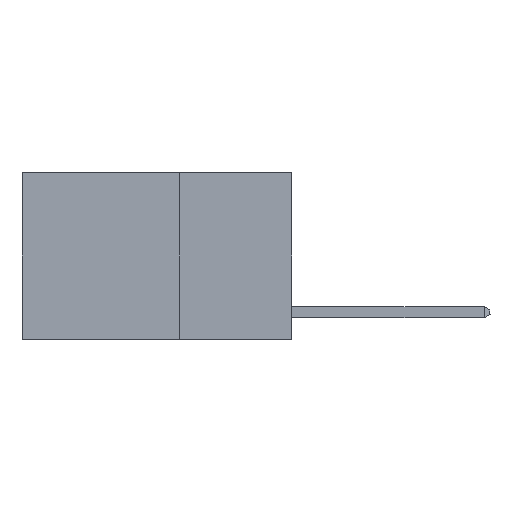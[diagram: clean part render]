
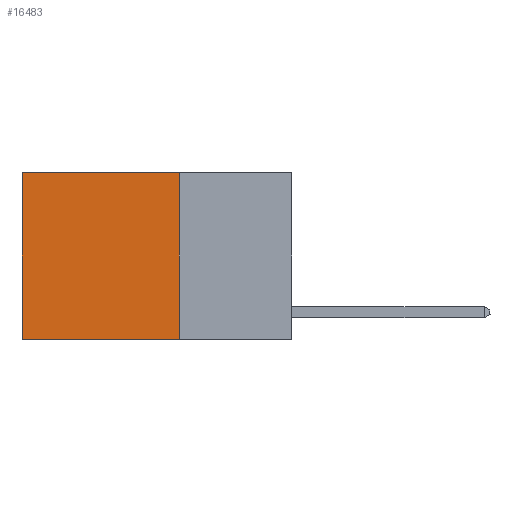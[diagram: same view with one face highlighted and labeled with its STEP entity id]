
A CAD part, left-side view. The second image highlights one B-rep face of the part: STEP entity #16483.
In plain terms, the highlighted planar face has unit normal (-1, 0, 0).
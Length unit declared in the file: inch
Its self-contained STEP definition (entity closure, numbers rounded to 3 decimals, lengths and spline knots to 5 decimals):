
#211 = DIRECTION ( 'NONE',  ( 0., 0., -1. ) ) ;
#755 = CARTESIAN_POINT ( 'NONE',  ( 0.2625, 0.25, -0.37 ) ) ;
#944 = CARTESIAN_POINT ( 'NONE',  ( 0.2625, 0.25, 0. ) ) ;
#2361 = LINE ( 'NONE', #10757, #10748 ) ;
#2517 = CARTESIAN_POINT ( 'NONE',  ( 0.2625, 0.25, 0. ) ) ;
#3203 = EDGE_CURVE ( 'NONE', #7254, #12237, #17413, .T. ) ;
#3739 = DIRECTION ( 'NONE',  ( 0., 0., -1. ) ) ;
#4208 = DIRECTION ( 'NONE',  ( 0., 0., -1. ) ) ;
#6625 = ORIENTED_EDGE ( 'NONE', *, *, #14745, .T. ) ;
#7254 = VERTEX_POINT ( 'NONE', #7407 ) ;
#7407 = CARTESIAN_POINT ( 'NONE',  ( 0.2625, 0.6, 0. ) ) ;
#8365 = VERTEX_POINT ( 'NONE', #944 ) ;
#8452 = VECTOR ( 'NONE', #14415, 39.37008 ) ;
#8497 = EDGE_LOOP ( 'NONE', ( #17888, #10391, #9834, #6625 ) ) ;
#9010 = VECTOR ( 'NONE', #3739, 39.37008 ) ;
#9834 = ORIENTED_EDGE ( 'NONE', *, *, #10853, .F. ) ;
#10391 = ORIENTED_EDGE ( 'NONE', *, *, #19052, .F. ) ;
#10748 = VECTOR ( 'NONE', #14100, 39.37008 ) ;
#10757 = CARTESIAN_POINT ( 'NONE',  ( 0.2625, 0.25, 0. ) ) ;
#10853 = EDGE_CURVE ( 'NONE', #8365, #15404, #19815, .T. ) ;
#11202 = FACE_OUTER_BOUND ( 'NONE', #8497, .T. ) ;
#12237 = VERTEX_POINT ( 'NONE', #15357 ) ;
#14100 = DIRECTION ( 'NONE',  ( 0., 1., 0. ) ) ;
#14223 = DIRECTION ( 'NONE',  ( 1., 0., 0. ) ) ;
#14415 = DIRECTION ( 'NONE',  ( 0., 1., 0. ) ) ;
#14745 = EDGE_CURVE ( 'NONE', #8365, #7254, #2361, .T. ) ;
#15357 = CARTESIAN_POINT ( 'NONE',  ( 0.2625, 0.6, -0.37 ) ) ;
#15404 = VERTEX_POINT ( 'NONE', #755 ) ;
#15450 = CARTESIAN_POINT ( 'NONE',  ( 0.2625, 0.6, 0. ) ) ;
#16483 = ADVANCED_FACE ( 'NONE', ( #11202 ), #20955, .F. ) ;
#17358 = LINE ( 'NONE', #19449, #8452 ) ;
#17413 = LINE ( 'NONE', #15450, #9010 ) ;
#17888 = ORIENTED_EDGE ( 'NONE', *, *, #3203, .T. ) ;
#18514 = AXIS2_PLACEMENT_3D ( 'NONE', #2517, #14223, #4208 ) ;
#19052 = EDGE_CURVE ( 'NONE', #15404, #12237, #17358, .T. ) ;
#19281 = VECTOR ( 'NONE', #211, 39.37008 ) ;
#19449 = CARTESIAN_POINT ( 'NONE',  ( 0.2625, 0.25, -0.37 ) ) ;
#19815 = LINE ( 'NONE', #20220, #19281 ) ;
#20220 = CARTESIAN_POINT ( 'NONE',  ( 0.2625, 0.25, 0. ) ) ;
#20955 = PLANE ( 'NONE',  #18514 ) ;
